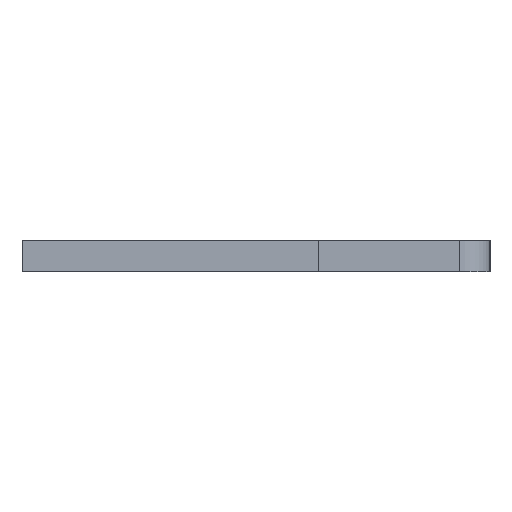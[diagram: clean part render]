
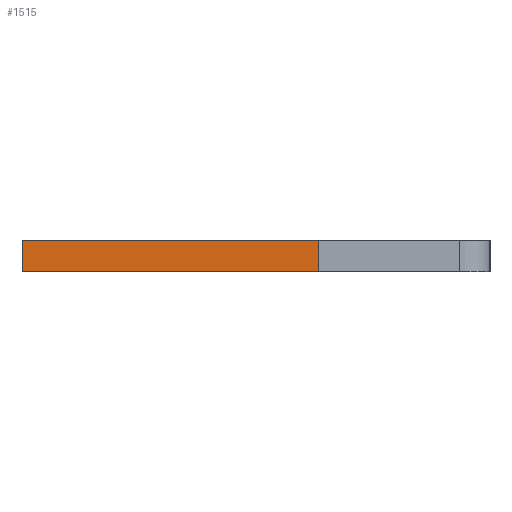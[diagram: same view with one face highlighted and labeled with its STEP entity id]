
A CAD part, left-side view. The second image highlights one B-rep face of the part: STEP entity #1515.
In plain terms, the highlighted face is planar.
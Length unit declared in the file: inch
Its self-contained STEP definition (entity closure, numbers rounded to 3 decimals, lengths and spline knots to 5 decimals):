
#2 = DIRECTION ( 'NONE',  ( 0., 0., 1. ) ) ;
#161 = CARTESIAN_POINT ( 'NONE',  ( -0.01, 0.15, -0.04 ) ) ;
#180 = CARTESIAN_POINT ( 'NONE',  ( 0.01, 0.15, -0.04 ) ) ;
#192 = EDGE_CURVE ( 'NONE', #1867, #1942, #1934, .T. ) ;
#196 = CARTESIAN_POINT ( 'NONE',  ( 0.01, 0.15, -0.04 ) ) ;
#315 = VECTOR ( 'NONE', #1941, 39.37008 ) ;
#325 = VERTEX_POINT ( 'NONE', #411 ) ;
#344 = VECTOR ( 'NONE', #1227, 39.37008 ) ;
#411 = CARTESIAN_POINT ( 'NONE',  ( 0.01, -0.04, -0.04 ) ) ;
#458 = ORIENTED_EDGE ( 'NONE', *, *, #534, .F. ) ;
#534 = EDGE_CURVE ( 'NONE', #325, #1101, #2153, .T. ) ;
#546 = ORIENTED_EDGE ( 'NONE', *, *, #1386, .F. ) ;
#715 = ORIENTED_EDGE ( 'NONE', *, *, #192, .T. ) ;
#744 = CARTESIAN_POINT ( 'NONE',  ( 0.01, 0.15, -0.04 ) ) ;
#860 = VECTOR ( 'NONE', #1437, 39.37008 ) ;
#881 = DIRECTION ( 'NONE',  ( -1., 0., 0. ) ) ;
#1076 = CARTESIAN_POINT ( 'NONE',  ( 0.01, 0.15, -0.04 ) ) ;
#1084 = CARTESIAN_POINT ( 'NONE',  ( 0.01, -0.04, -0.04 ) ) ;
#1101 = VERTEX_POINT ( 'NONE', #180 ) ;
#1115 = CARTESIAN_POINT ( 'NONE',  ( -0.01, -0.04, -0.04 ) ) ;
#1227 = DIRECTION ( 'NONE',  ( 0., 1., 0. ) ) ;
#1306 = ORIENTED_EDGE ( 'NONE', *, *, #1567, .T. ) ;
#1386 = EDGE_CURVE ( 'NONE', #1101, #1942, #1516, .T. ) ;
#1400 = DIRECTION ( 'NONE',  ( 1., 0., 0. ) ) ;
#1437 = DIRECTION ( 'NONE',  ( 0., 1., 0. ) ) ;
#1515 = ADVANCED_FACE ( 'NONE', ( #1836 ), #1777, .F. ) ;
#1516 = LINE ( 'NONE', #1076, #315 ) ;
#1567 = EDGE_CURVE ( 'NONE', #325, #1867, #2039, .T. ) ;
#1762 = EDGE_LOOP ( 'NONE', ( #715, #546, #458, #1306 ) ) ;
#1777 = PLANE ( 'NONE',  #1823 ) ;
#1823 = AXIS2_PLACEMENT_3D ( 'NONE', #744, #2, #1400 ) ;
#1836 = FACE_OUTER_BOUND ( 'NONE', #1762, .T. ) ;
#1863 = VECTOR ( 'NONE', #881, 39.37008 ) ;
#1867 = VERTEX_POINT ( 'NONE', #1115 ) ;
#1934 = LINE ( 'NONE', #161, #344 ) ;
#1941 = DIRECTION ( 'NONE',  ( -1., 0., 0. ) ) ;
#1942 = VERTEX_POINT ( 'NONE', #2134 ) ;
#2039 = LINE ( 'NONE', #1084, #1863 ) ;
#2134 = CARTESIAN_POINT ( 'NONE',  ( -0.01, 0.15, -0.04 ) ) ;
#2153 = LINE ( 'NONE', #196, #860 ) ;
